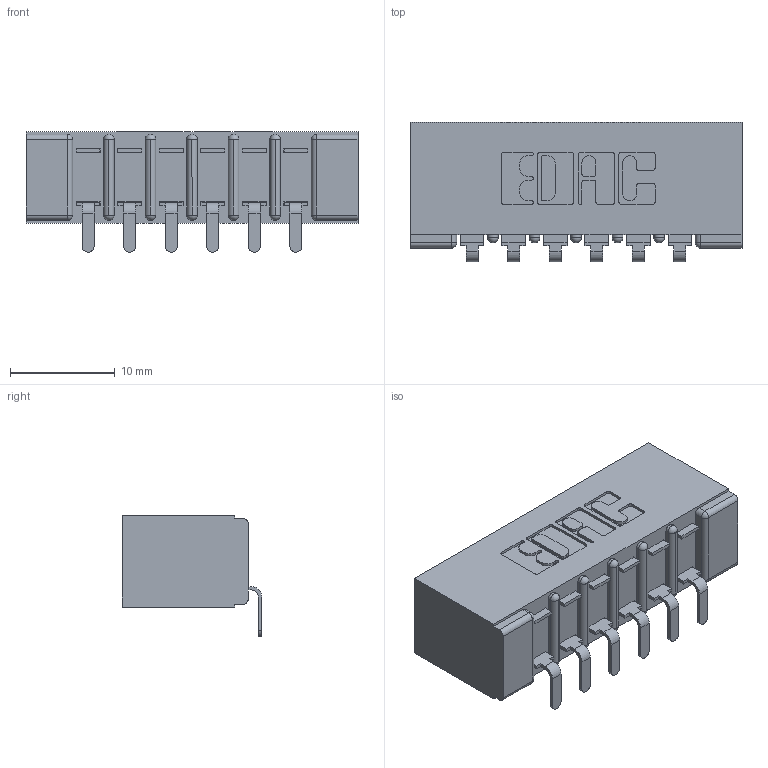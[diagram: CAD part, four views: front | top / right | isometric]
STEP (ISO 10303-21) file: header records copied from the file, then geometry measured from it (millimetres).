
FILE_DESCRIPTION (( 'STEP AP203' ), '1' );
FILE_NAME ('357-006-553-101.STEP', '2018-08-06T23:15:14', ( '' ), ( '' ), 'SwSTEP 2.0', 'SolidWorks 2016', '' );
FILE_SCHEMA (( 'CONFIG_CONTROL_DESIGN' ));
Length unit declared in the file: inch
Products named in the file (3): 307 Part_No Mounting Lugs; 307-290-002_553; 357-006-553-101
Assembly tree (7 placements, depth 2):
  357-006-553-101
    307 Part_No Mounting Lugs
    307-290-002_553  x6
Bounding box: 31.65 x 13.32 x 11.51 mm (x, y, z)
Volume: 2323.3 mm3; surface area: 3845 mm2
Topology: 7 solids, 7 shells, 585 faces, 1763 edges, 1154 vertices
Faces by surface type: plane 348, cylinder 223, sphere 14
Entity records: 10158 total; most frequent: CARTESIAN_POINT 1708, ORIENTED_EDGE 1698, DIRECTION 1675, EDGE_CURVE 849, LINE 633, VECTOR 633, VERTEX_POINT 554, AXIS2_PLACEMENT_3D 521
